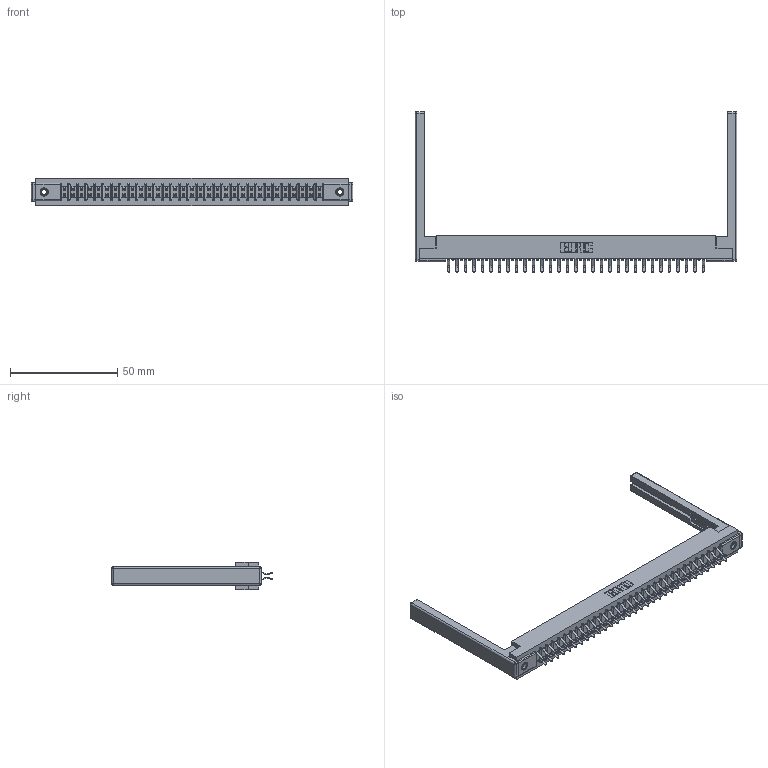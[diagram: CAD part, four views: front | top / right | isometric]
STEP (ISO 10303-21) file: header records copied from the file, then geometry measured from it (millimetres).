
FILE_DESCRIPTION (( 'STEP AP203' ), '1' );
FILE_NAME ('307-062-556-268.STEP', '2019-09-06T16:18:56', ( '' ), ( '' ), 'SwSTEP 2.0', 'SolidWorks 2016', '' );
FILE_SCHEMA (( 'CONFIG_CONTROL_DESIGN' ));
Length unit declared in the file: inch
Products named in the file (5): 307-220-068; 307-062-556-268; 307 Part_.156 Dia Mounting Holes; 307-290-001_556; 345-250-001_345-250-001-102
Assembly tree (67 placements, depth 2):
  307-062-556-268
    307 Part_.156 Dia Mounting Holes
    307-290-001_556  x62
    307-220-068  x2
    345-250-001_345-250-001-102  x2
Bounding box: 150.27 x 74.93 x 12.7 mm (x, y, z)
Volume: 20270.5 mm3; surface area: 23038.8 mm2
Topology: 67 solids, 67 shells, 3404 faces, 9517 edges, 6154 vertices
Faces by surface type: plane 2204, cylinder 1112, sphere 72, cone 12, torus 4
Entity records: 31787 total; most frequent: CARTESIAN_POINT 5180, ORIENTED_EDGE 5124, DIRECTION 5094, EDGE_CURVE 2562, LINE 1958, VECTOR 1958, VERTEX_POINT 1654, AXIS2_PLACEMENT_3D 1568
